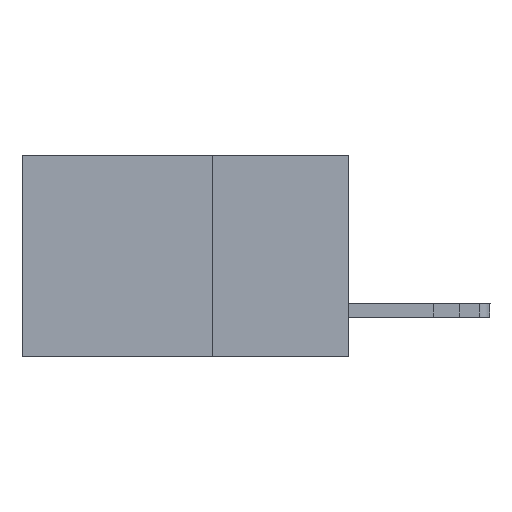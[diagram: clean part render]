
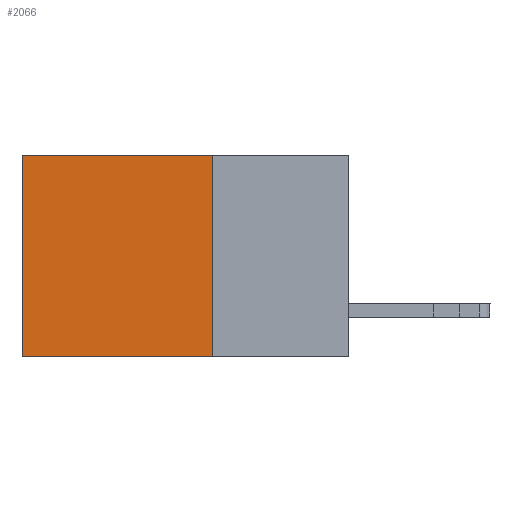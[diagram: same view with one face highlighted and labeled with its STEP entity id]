
A CAD part, left-side view. The second image highlights one B-rep face of the part: STEP entity #2066.
In plain terms, the highlighted planar face has unit normal (-1, 0, 0).
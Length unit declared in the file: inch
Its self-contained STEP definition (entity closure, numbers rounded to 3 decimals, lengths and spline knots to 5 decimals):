
#27 = CARTESIAN_POINT ( 'NONE',  ( 0.298, 0.25, -0.37 ) ) ;
#75 = EDGE_CURVE ( 'NONE', #11374, #3615, #3953, .T. ) ;
#96 = ORIENTED_EDGE ( 'NONE', *, *, #2521, .F. ) ;
#1475 = VECTOR ( 'NONE', #9653, 39.37008 ) ;
#1500 = CARTESIAN_POINT ( 'NONE',  ( 0.298, 0.25, 0. ) ) ;
#1829 = CARTESIAN_POINT ( 'NONE',  ( 0.298, 0.6, 0. ) ) ;
#2066 = ADVANCED_FACE ( 'NONE', ( #5134 ), #10652, .F. ) ;
#2521 = EDGE_CURVE ( 'NONE', #10549, #3615, #3088, .T. ) ;
#3073 = VECTOR ( 'NONE', #10881, 39.37008 ) ;
#3088 = LINE ( 'NONE', #27, #7287 ) ;
#3615 = VERTEX_POINT ( 'NONE', #6692 ) ;
#3953 = LINE ( 'NONE', #13599, #12157 ) ;
#4256 = ORIENTED_EDGE ( 'NONE', *, *, #10855, .F. ) ;
#4271 = DIRECTION ( 'NONE',  ( 1., 0., 0. ) ) ;
#4321 = DIRECTION ( 'NONE',  ( 0., 0., -1. ) ) ;
#5053 = DIRECTION ( 'NONE',  ( 0., 0., -1. ) ) ;
#5134 = FACE_OUTER_BOUND ( 'NONE', #13973, .T. ) ;
#5311 = CARTESIAN_POINT ( 'NONE',  ( 0.298, 0.25, -0.37 ) ) ;
#6345 = LINE ( 'NONE', #11798, #1475 ) ;
#6692 = CARTESIAN_POINT ( 'NONE',  ( 0.298, 0.6, -0.37 ) ) ;
#7287 = VECTOR ( 'NONE', #11708, 39.37008 ) ;
#8141 = EDGE_CURVE ( 'NONE', #12079, #11374, #6345, .T. ) ;
#9653 = DIRECTION ( 'NONE',  ( 0., 1., 0. ) ) ;
#9717 = AXIS2_PLACEMENT_3D ( 'NONE', #11893, #4271, #4321 ) ;
#10549 = VERTEX_POINT ( 'NONE', #5311 ) ;
#10652 = PLANE ( 'NONE',  #9717 ) ;
#10758 = ORIENTED_EDGE ( 'NONE', *, *, #75, .T. ) ;
#10855 = EDGE_CURVE ( 'NONE', #12079, #10549, #11975, .T. ) ;
#10881 = DIRECTION ( 'NONE',  ( 0., 0., -1. ) ) ;
#11374 = VERTEX_POINT ( 'NONE', #1829 ) ;
#11708 = DIRECTION ( 'NONE',  ( 0., 1., 0. ) ) ;
#11798 = CARTESIAN_POINT ( 'NONE',  ( 0.298, 0.25, 0. ) ) ;
#11893 = CARTESIAN_POINT ( 'NONE',  ( 0.298, 0.25, 0. ) ) ;
#11975 = LINE ( 'NONE', #13138, #3073 ) ;
#12079 = VERTEX_POINT ( 'NONE', #1500 ) ;
#12157 = VECTOR ( 'NONE', #5053, 39.37008 ) ;
#13138 = CARTESIAN_POINT ( 'NONE',  ( 0.298, 0.25, 0. ) ) ;
#13458 = ORIENTED_EDGE ( 'NONE', *, *, #8141, .T. ) ;
#13599 = CARTESIAN_POINT ( 'NONE',  ( 0.298, 0.6, 0. ) ) ;
#13973 = EDGE_LOOP ( 'NONE', ( #10758, #96, #4256, #13458 ) ) ;
